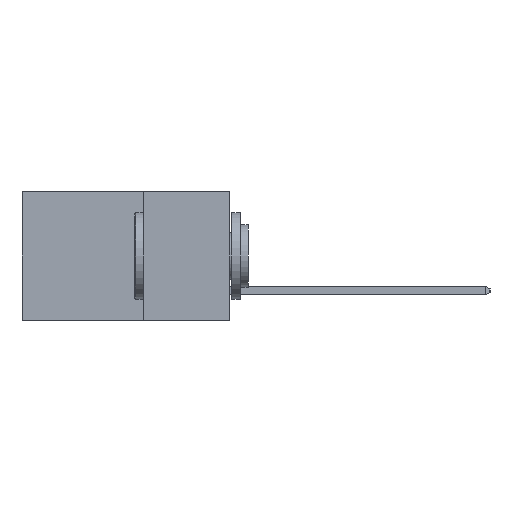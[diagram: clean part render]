
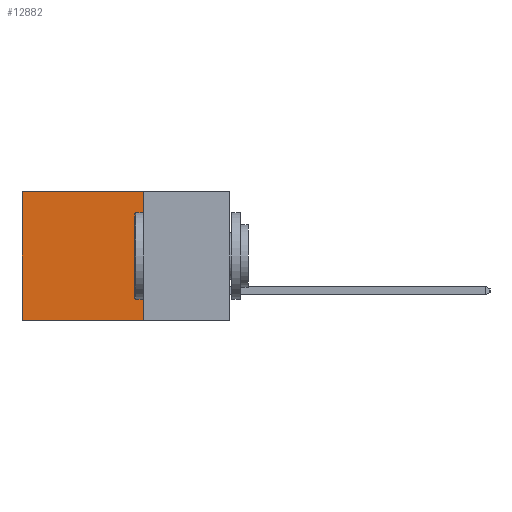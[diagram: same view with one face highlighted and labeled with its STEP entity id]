
A CAD part, left-side view. The second image highlights one B-rep face of the part: STEP entity #12882.
In plain terms, the highlighted planar face has unit normal (-1, 0, 0).
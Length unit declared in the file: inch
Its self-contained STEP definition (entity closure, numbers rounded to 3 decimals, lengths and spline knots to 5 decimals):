
#93 = LINE ( 'NONE', #16564, #16048 ) ;
#444 = VECTOR ( 'NONE', #9128, 39.37008 ) ;
#885 = EDGE_CURVE ( 'NONE', #7979, #1964, #93, .T. ) ;
#1964 = VERTEX_POINT ( 'NONE', #11918 ) ;
#2073 = EDGE_LOOP ( 'NONE', ( #11973, #18925, #5635, #6337 ) ) ;
#2314 = CARTESIAN_POINT ( 'NONE',  ( 0.298, 0.25, 0. ) ) ;
#3089 = EDGE_CURVE ( 'NONE', #12201, #25389, #11609, .T. ) ;
#4507 = DIRECTION ( 'NONE',  ( 0., 0., -1. ) ) ;
#4584 = EDGE_CURVE ( 'NONE', #12201, #7979, #23051, .T. ) ;
#5635 = ORIENTED_EDGE ( 'NONE', *, *, #4584, .F. ) ;
#6337 = ORIENTED_EDGE ( 'NONE', *, *, #3089, .T. ) ;
#6386 = LINE ( 'NONE', #22544, #21840 ) ;
#7282 = DIRECTION ( 'NONE',  ( 0., 0., -1. ) ) ;
#7979 = VERTEX_POINT ( 'NONE', #20374 ) ;
#9128 = DIRECTION ( 'NONE',  ( 0., 1., 0. ) ) ;
#11609 = LINE ( 'NONE', #2314, #444 ) ;
#11918 = CARTESIAN_POINT ( 'NONE',  ( 0.298, 0.6, -0.37 ) ) ;
#11959 = AXIS2_PLACEMENT_3D ( 'NONE', #22624, #16783, #4507 ) ;
#11973 = ORIENTED_EDGE ( 'NONE', *, *, #12831, .T. ) ;
#12201 = VERTEX_POINT ( 'NONE', #24031 ) ;
#12831 = EDGE_CURVE ( 'NONE', #25389, #1964, #6386, .T. ) ;
#12882 = ADVANCED_FACE ( 'NONE', ( #15964 ), #16699, .F. ) ;
#15964 = FACE_OUTER_BOUND ( 'NONE', #2073, .T. ) ;
#16048 = VECTOR ( 'NONE', #19116, 39.37008 ) ;
#16564 = CARTESIAN_POINT ( 'NONE',  ( 0.298, 0.25, -0.37 ) ) ;
#16699 = PLANE ( 'NONE',  #11959 ) ;
#16783 = DIRECTION ( 'NONE',  ( 1., 0., 0. ) ) ;
#16931 = CARTESIAN_POINT ( 'NONE',  ( 0.298, 0.25, 0. ) ) ;
#18925 = ORIENTED_EDGE ( 'NONE', *, *, #885, .F. ) ;
#19116 = DIRECTION ( 'NONE',  ( 0., 1., 0. ) ) ;
#20374 = CARTESIAN_POINT ( 'NONE',  ( 0.298, 0.25, -0.37 ) ) ;
#21840 = VECTOR ( 'NONE', #24470, 39.37008 ) ;
#22475 = VECTOR ( 'NONE', #7282, 39.37008 ) ;
#22544 = CARTESIAN_POINT ( 'NONE',  ( 0.298, 0.6, 0. ) ) ;
#22624 = CARTESIAN_POINT ( 'NONE',  ( 0.298, 0.25, 0. ) ) ;
#22635 = CARTESIAN_POINT ( 'NONE',  ( 0.298, 0.6, 0. ) ) ;
#23051 = LINE ( 'NONE', #16931, #22475 ) ;
#24031 = CARTESIAN_POINT ( 'NONE',  ( 0.298, 0.25, 0. ) ) ;
#24470 = DIRECTION ( 'NONE',  ( 0., 0., -1. ) ) ;
#25389 = VERTEX_POINT ( 'NONE', #22635 ) ;
